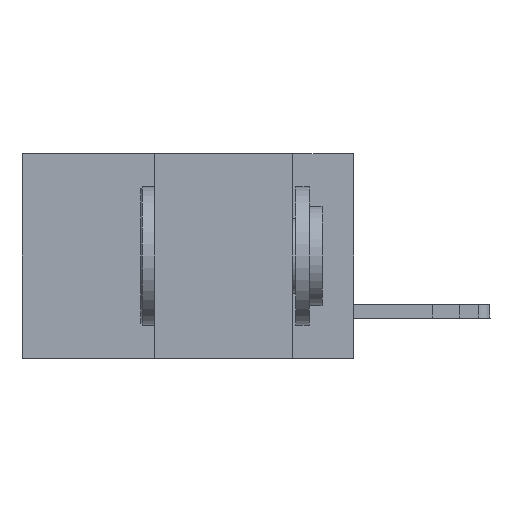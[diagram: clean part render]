
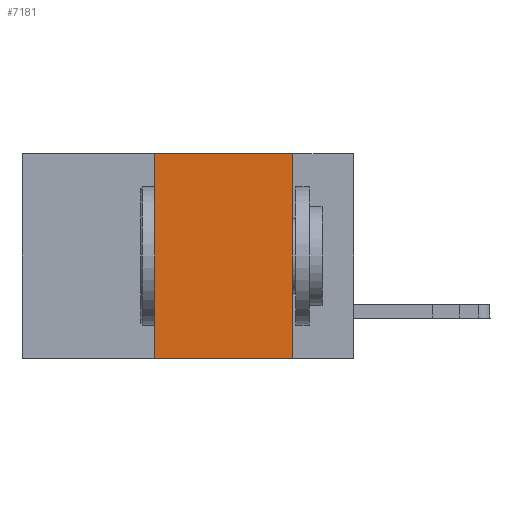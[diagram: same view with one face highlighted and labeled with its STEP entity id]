
A CAD part, left-side view. The second image highlights one B-rep face of the part: STEP entity #7181.
In plain terms, the highlighted planar face has unit normal (-1, 0, 0).
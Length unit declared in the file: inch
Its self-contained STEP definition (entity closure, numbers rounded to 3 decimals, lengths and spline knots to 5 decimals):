
#3 = EDGE_CURVE ( 'NONE', #28830, #21008, #26814, .T. ) ;
#750 = VERTEX_POINT ( 'NONE', #21820 ) ;
#1145 = ORIENTED_EDGE ( 'NONE', *, *, #3, .F. ) ;
#1875 = EDGE_CURVE ( 'NONE', #21008, #750, #20020, .T. ) ;
#2129 = CARTESIAN_POINT ( 'NONE',  ( 0., 0.6, 0. ) ) ;
#2304 = PLANE ( 'NONE',  #24739 ) ;
#3245 = ORIENTED_EDGE ( 'NONE', *, *, #17616, .T. ) ;
#6711 = DIRECTION ( 'NONE',  ( 0., 0., -1. ) ) ;
#7181 = ADVANCED_FACE ( 'NONE', ( #20453 ), #2304, .F. ) ;
#7669 = EDGE_CURVE ( 'NONE', #11105, #28830, #16547, .T. ) ;
#8268 = LINE ( 'NONE', #15356, #23495 ) ;
#8942 = EDGE_LOOP ( 'NONE', ( #33133, #1145, #14600, #3245 ) ) ;
#9884 = VECTOR ( 'NONE', #6711, 39.37008 ) ;
#11105 = VERTEX_POINT ( 'NONE', #31845 ) ;
#13404 = VECTOR ( 'NONE', #24740, 39.37008 ) ;
#14600 = ORIENTED_EDGE ( 'NONE', *, *, #7669, .F. ) ;
#15356 = CARTESIAN_POINT ( 'NONE',  ( 0., 0.6, -0.37 ) ) ;
#16547 = LINE ( 'NONE', #32440, #25846 ) ;
#17616 = EDGE_CURVE ( 'NONE', #11105, #750, #8268, .T. ) ;
#19850 = CARTESIAN_POINT ( 'NONE',  ( 0., 0.11, 0. ) ) ;
#20020 = LINE ( 'NONE', #19850, #9884 ) ;
#20453 = FACE_OUTER_BOUND ( 'NONE', #8942, .T. ) ;
#21008 = VERTEX_POINT ( 'NONE', #31354 ) ;
#21820 = CARTESIAN_POINT ( 'NONE',  ( 0., 0.11, -0.37 ) ) ;
#23495 = VECTOR ( 'NONE', #28994, 39.37008 ) ;
#24739 = AXIS2_PLACEMENT_3D ( 'NONE', #2129, #31001, #28573 ) ;
#24740 = DIRECTION ( 'NONE',  ( 0., -1., 0. ) ) ;
#24861 = DIRECTION ( 'NONE',  ( 0., 0., 1. ) ) ;
#25846 = VECTOR ( 'NONE', #24861, 39.37008 ) ;
#26814 = LINE ( 'NONE', #29926, #13404 ) ;
#28573 = DIRECTION ( 'NONE',  ( 0., 0., -1. ) ) ;
#28830 = VERTEX_POINT ( 'NONE', #32734 ) ;
#28994 = DIRECTION ( 'NONE',  ( 0., -1., 0. ) ) ;
#29926 = CARTESIAN_POINT ( 'NONE',  ( 0., 0.6, 0. ) ) ;
#31001 = DIRECTION ( 'NONE',  ( 1., 0., 0. ) ) ;
#31354 = CARTESIAN_POINT ( 'NONE',  ( 0., 0.11, 0. ) ) ;
#31845 = CARTESIAN_POINT ( 'NONE',  ( 0., 0.36, -0.37 ) ) ;
#32440 = CARTESIAN_POINT ( 'NONE',  ( 0., 0.36, 0. ) ) ;
#32734 = CARTESIAN_POINT ( 'NONE',  ( 0., 0.36, 0. ) ) ;
#33133 = ORIENTED_EDGE ( 'NONE', *, *, #1875, .F. ) ;
